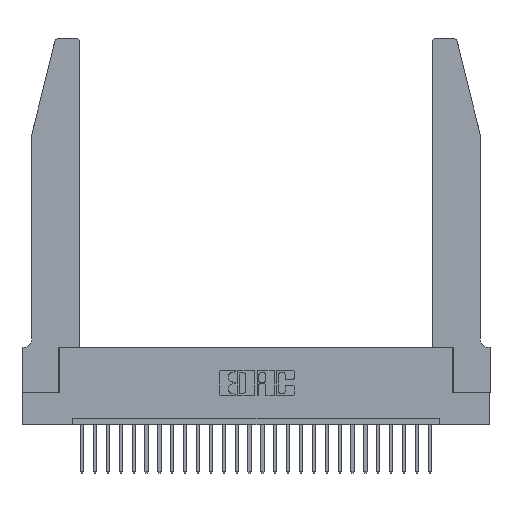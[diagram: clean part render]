
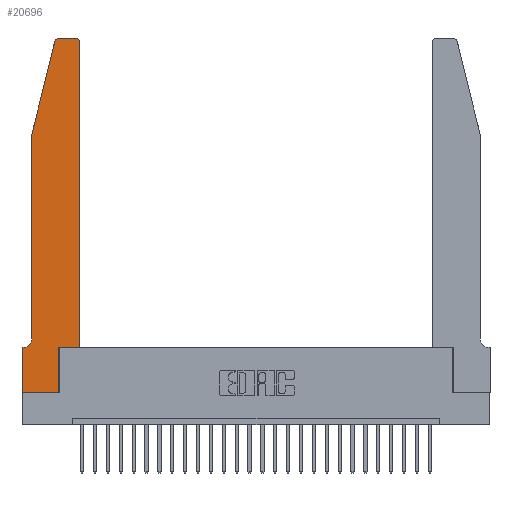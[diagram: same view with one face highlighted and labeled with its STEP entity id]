
A CAD part, top view. The second image highlights one B-rep face of the part: STEP entity #20696.
In plain terms, the highlighted planar face has unit normal (0, 0, 1).
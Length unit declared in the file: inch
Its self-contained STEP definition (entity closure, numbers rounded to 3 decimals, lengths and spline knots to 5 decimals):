
#695 = ORIENTED_EDGE ( 'NONE', *, *, #17412, .T. ) ;
#1105 = VECTOR ( 'NONE', #3596, 39.37008 ) ;
#1186 = VECTOR ( 'NONE', #2191, 39.37008 ) ;
#1480 = CIRCLE ( 'NONE', #11325, 0.03 ) ;
#1887 = LINE ( 'NONE', #16457, #22603 ) ;
#1946 = LINE ( 'NONE', #15449, #23992 ) ;
#2191 = DIRECTION ( 'NONE',  ( 0., -1., 0. ) ) ;
#3207 = LINE ( 'NONE', #15015, #1186 ) ;
#3297 = EDGE_CURVE ( 'NONE', #15321, #19397, #3207, .T. ) ;
#3457 = ORIENTED_EDGE ( 'NONE', *, *, #19065, .T. ) ;
#3586 = ORIENTED_EDGE ( 'NONE', *, *, #7357, .T. ) ;
#3596 = DIRECTION ( 'NONE',  ( -0.239, -0.971, 0. ) ) ;
#3746 = VECTOR ( 'NONE', #20542, 39.37008 ) ;
#3910 = DIRECTION ( 'NONE',  ( -1., 0., 0. ) ) ;
#4453 = LINE ( 'NONE', #11128, #26210 ) ;
#4684 = CARTESIAN_POINT ( 'NONE',  ( 0.25487, 2.72718, 0.37 ) ) ;
#5163 = CARTESIAN_POINT ( 'NONE',  ( 0.284, 2.75, 0.37 ) ) ;
#5371 = VECTOR ( 'NONE', #5501, 39.37008 ) ;
#5501 = DIRECTION ( 'NONE',  ( 0., 1., 0. ) ) ;
#5609 = DIRECTION ( 'NONE',  ( 1., 0., 0. ) ) ;
#5873 = EDGE_CURVE ( 'NONE', #26363, #18848, #18564, .T. ) ;
#6019 = ORIENTED_EDGE ( 'NONE', *, *, #20331, .T. ) ;
#6089 = CARTESIAN_POINT ( 'NONE',  ( 0.4205, 2.75, 0.37 ) ) ;
#6164 = CARTESIAN_POINT ( 'NONE',  ( 0.4505, 0.35, 0.37 ) ) ;
#6289 = VERTEX_POINT ( 'NONE', #5163 ) ;
#6326 = CARTESIAN_POINT ( 'NONE',  ( 0.0055, 0.42, 0.37 ) ) ;
#6486 = VERTEX_POINT ( 'NONE', #17802 ) ;
#6557 = ORIENTED_EDGE ( 'NONE', *, *, #23842, .T. ) ;
#7183 = VERTEX_POINT ( 'NONE', #13329 ) ;
#7233 = EDGE_LOOP ( 'NONE', ( #17714, #6019, #9303, #27259, #8346, #8404, #13660, #3586, #6557, #9557, #3457, #695 ) ) ;
#7357 = EDGE_CURVE ( 'NONE', #7183, #26753, #20496, .T. ) ;
#7644 = CARTESIAN_POINT ( 'NONE',  ( 0., 0.35, 0.37 ) ) ;
#7827 = CARTESIAN_POINT ( 'NONE',  ( 0., 0., 0.37 ) ) ;
#8346 = ORIENTED_EDGE ( 'NONE', *, *, #18900, .T. ) ;
#8368 = DIRECTION ( 'NONE',  ( -1., 0., 0. ) ) ;
#8404 = ORIENTED_EDGE ( 'NONE', *, *, #5873, .T. ) ;
#9303 = ORIENTED_EDGE ( 'NONE', *, *, #23605, .T. ) ;
#9339 = DIRECTION ( 'NONE',  ( 0., 0., 1. ) ) ;
#9374 = AXIS2_PLACEMENT_3D ( 'NONE', #9988, #24862, #5609 ) ;
#9557 = ORIENTED_EDGE ( 'NONE', *, *, #12964, .T. ) ;
#9988 = CARTESIAN_POINT ( 'NONE',  ( 0.284, 2.72, 0.37 ) ) ;
#10014 = VERTEX_POINT ( 'NONE', #6089 ) ;
#11049 = LINE ( 'NONE', #13915, #5371 ) ;
#11128 = CARTESIAN_POINT ( 'NONE',  ( 0.2865, 0.35, 0.37 ) ) ;
#11209 = DIRECTION ( 'NONE',  ( -1., 0., 0. ) ) ;
#11325 = AXIS2_PLACEMENT_3D ( 'NONE', #27204, #20941, #18604 ) ;
#12342 = DIRECTION ( 'NONE',  ( 0., -1., 0. ) ) ;
#12503 = VERTEX_POINT ( 'NONE', #18196 ) ;
#12886 = VECTOR ( 'NONE', #8368, 39.37008 ) ;
#12964 = EDGE_CURVE ( 'NONE', #26063, #12503, #27142, .T. ) ;
#13176 = LINE ( 'NONE', #25401, #1105 ) ;
#13329 = CARTESIAN_POINT ( 'NONE',  ( 0., 0., 0.37 ) ) ;
#13660 = ORIENTED_EDGE ( 'NONE', *, *, #27706, .T. ) ;
#13915 = CARTESIAN_POINT ( 'NONE',  ( 0.4505, 0.35, 0.37 ) ) ;
#14079 = VECTOR ( 'NONE', #16568, 39.37008 ) ;
#15015 = CARTESIAN_POINT ( 'NONE',  ( 0.0755, 2., 0.37 ) ) ;
#15124 = CARTESIAN_POINT ( 'NONE',  ( 0.2865, 0.35, 0.37 ) ) ;
#15321 = VERTEX_POINT ( 'NONE', #17960 ) ;
#15449 = CARTESIAN_POINT ( 'NONE',  ( 0.2605, 2.75, 0.37 ) ) ;
#15852 = AXIS2_PLACEMENT_3D ( 'NONE', #6326, #18568, #3910 ) ;
#16457 = CARTESIAN_POINT ( 'NONE',  ( 0., 0., 0.37 ) ) ;
#16568 = DIRECTION ( 'NONE',  ( 1., 0., 0. ) ) ;
#16923 = VERTEX_POINT ( 'NONE', #4684 ) ;
#17344 = DIRECTION ( 'NONE',  ( 0., 1., 0. ) ) ;
#17412 = EDGE_CURVE ( 'NONE', #6486, #10014, #1480, .T. ) ;
#17714 = ORIENTED_EDGE ( 'NONE', *, *, #26911, .T. ) ;
#17716 = FACE_OUTER_BOUND ( 'NONE', #7233, .T. ) ;
#17802 = CARTESIAN_POINT ( 'NONE',  ( 0.4505, 2.72, 0.37 ) ) ;
#17960 = CARTESIAN_POINT ( 'NONE',  ( 0.0755, 2., 0.37 ) ) ;
#18196 = CARTESIAN_POINT ( 'NONE',  ( 0.4505, 0.35, 0.37 ) ) ;
#18564 = LINE ( 'NONE', #21265, #12886 ) ;
#18568 = DIRECTION ( 'NONE',  ( 0., 0., -1. ) ) ;
#18604 = DIRECTION ( 'NONE',  ( 1., 0., 0. ) ) ;
#18804 = CIRCLE ( 'NONE', #15852, 0.07 ) ;
#18848 = VERTEX_POINT ( 'NONE', #7644 ) ;
#18900 = EDGE_CURVE ( 'NONE', #19397, #26363, #18804, .T. ) ;
#19065 = EDGE_CURVE ( 'NONE', #12503, #6486, #11049, .T. ) ;
#19397 = VERTEX_POINT ( 'NONE', #25312 ) ;
#19489 = CARTESIAN_POINT ( 'NONE',  ( 0.2865, 0., 0.37 ) ) ;
#19628 = AXIS2_PLACEMENT_3D ( 'NONE', #22178, #9339, #24498 ) ;
#20227 = PLANE ( 'NONE',  #19628 ) ;
#20331 = EDGE_CURVE ( 'NONE', #6289, #16923, #20756, .T. ) ;
#20496 = LINE ( 'NONE', #7827, #3746 ) ;
#20542 = DIRECTION ( 'NONE',  ( 1., 0., 0. ) ) ;
#20696 = ADVANCED_FACE ( 'NONE', ( #17716 ), #20227, .T. ) ;
#20756 = CIRCLE ( 'NONE', #9374, 0.03 ) ;
#20941 = DIRECTION ( 'NONE',  ( 0., 0., 1. ) ) ;
#21265 = CARTESIAN_POINT ( 'NONE',  ( 0.0755, 0.35, 0.37 ) ) ;
#22178 = CARTESIAN_POINT ( 'NONE',  ( 0., 0.35, 0.37 ) ) ;
#22603 = VECTOR ( 'NONE', #12342, 39.37008 ) ;
#23605 = EDGE_CURVE ( 'NONE', #16923, #15321, #13176, .T. ) ;
#23842 = EDGE_CURVE ( 'NONE', #26753, #26063, #4453, .T. ) ;
#23992 = VECTOR ( 'NONE', #11209, 39.37008 ) ;
#24498 = DIRECTION ( 'NONE',  ( 1., 0., 0. ) ) ;
#24862 = DIRECTION ( 'NONE',  ( 0., 0., 1. ) ) ;
#25312 = CARTESIAN_POINT ( 'NONE',  ( 0.0755, 0.42, 0.37 ) ) ;
#25401 = CARTESIAN_POINT ( 'NONE',  ( 0.0755, 2., 0.37 ) ) ;
#26063 = VERTEX_POINT ( 'NONE', #15124 ) ;
#26210 = VECTOR ( 'NONE', #17344, 39.37008 ) ;
#26363 = VERTEX_POINT ( 'NONE', #26388 ) ;
#26388 = CARTESIAN_POINT ( 'NONE',  ( 0.0055, 0.35, 0.37 ) ) ;
#26753 = VERTEX_POINT ( 'NONE', #19489 ) ;
#26911 = EDGE_CURVE ( 'NONE', #10014, #6289, #1946, .T. ) ;
#27142 = LINE ( 'NONE', #6164, #14079 ) ;
#27204 = CARTESIAN_POINT ( 'NONE',  ( 0.4205, 2.72, 0.37 ) ) ;
#27259 = ORIENTED_EDGE ( 'NONE', *, *, #3297, .T. ) ;
#27706 = EDGE_CURVE ( 'NONE', #18848, #7183, #1887, .T. ) ;
